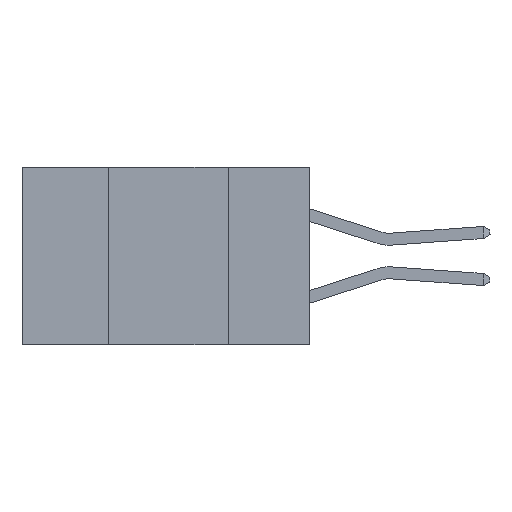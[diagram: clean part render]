
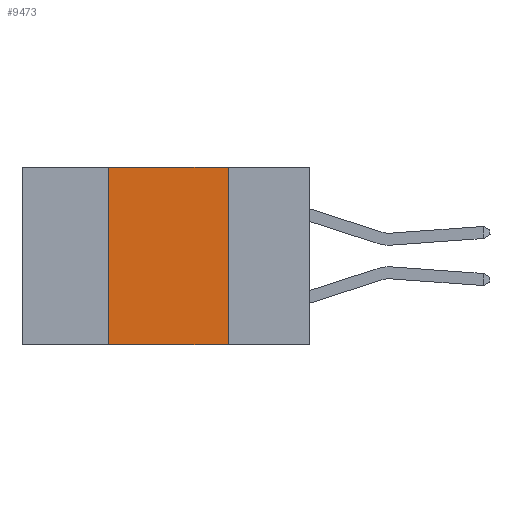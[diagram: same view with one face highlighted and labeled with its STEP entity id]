
A CAD part, left-side view. The second image highlights one B-rep face of the part: STEP entity #9473.
In plain terms, the highlighted planar face has unit normal (-1, 0, 0).
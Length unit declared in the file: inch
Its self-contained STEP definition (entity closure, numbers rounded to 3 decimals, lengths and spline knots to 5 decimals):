
#1128 = VECTOR ( 'NONE', #13885, 39.37008 ) ;
#2128 = CARTESIAN_POINT ( 'NONE',  ( 0., 0.6, 0. ) ) ;
#2676 = DIRECTION ( 'NONE',  ( 0., -1., 0. ) ) ;
#3066 = CARTESIAN_POINT ( 'NONE',  ( 0., 0.6, 0. ) ) ;
#3781 = VERTEX_POINT ( 'NONE', #9034 ) ;
#5067 = FACE_OUTER_BOUND ( 'NONE', #28267, .T. ) ;
#5304 = VERTEX_POINT ( 'NONE', #15495 ) ;
#5627 = LINE ( 'NONE', #27259, #1128 ) ;
#6877 = DIRECTION ( 'NONE',  ( 1., 0., 0. ) ) ;
#7494 = LINE ( 'NONE', #3066, #9199 ) ;
#9034 = CARTESIAN_POINT ( 'NONE',  ( 0., 0.42, 0. ) ) ;
#9103 = CARTESIAN_POINT ( 'NONE',  ( 0., 0.17, 0. ) ) ;
#9199 = VECTOR ( 'NONE', #2676, 39.37008 ) ;
#9473 = ADVANCED_FACE ( 'NONE', ( #5067 ), #11490, .F. ) ;
#10404 = ORIENTED_EDGE ( 'NONE', *, *, #20025, .F. ) ;
#11490 = PLANE ( 'NONE',  #12974 ) ;
#12974 = AXIS2_PLACEMENT_3D ( 'NONE', #2128, #6877, #27038 ) ;
#13355 = LINE ( 'NONE', #9103, #26652 ) ;
#13885 = DIRECTION ( 'NONE',  ( 0., 0., 1. ) ) ;
#15495 = CARTESIAN_POINT ( 'NONE',  ( 0., 0.17, 0. ) ) ;
#18229 = EDGE_CURVE ( 'NONE', #3781, #5304, #7494, .T. ) ;
#18566 = LINE ( 'NONE', #24984, #23104 ) ;
#18690 = CARTESIAN_POINT ( 'NONE',  ( 0., 0.42, -0.37 ) ) ;
#18748 = ORIENTED_EDGE ( 'NONE', *, *, #18229, .F. ) ;
#19808 = CARTESIAN_POINT ( 'NONE',  ( 0., 0.17, -0.37 ) ) ;
#20025 = EDGE_CURVE ( 'NONE', #5304, #22705, #13355, .T. ) ;
#22705 = VERTEX_POINT ( 'NONE', #19808 ) ;
#22988 = EDGE_CURVE ( 'NONE', #24951, #22705, #18566, .T. ) ;
#23104 = VECTOR ( 'NONE', #25170, 39.37008 ) ;
#23361 = EDGE_CURVE ( 'NONE', #24951, #3781, #5627, .T. ) ;
#24951 = VERTEX_POINT ( 'NONE', #18690 ) ;
#24984 = CARTESIAN_POINT ( 'NONE',  ( 0., 0.6, -0.37 ) ) ;
#25115 = ORIENTED_EDGE ( 'NONE', *, *, #22988, .T. ) ;
#25170 = DIRECTION ( 'NONE',  ( 0., -1., 0. ) ) ;
#26148 = ORIENTED_EDGE ( 'NONE', *, *, #23361, .F. ) ;
#26652 = VECTOR ( 'NONE', #26739, 39.37008 ) ;
#26739 = DIRECTION ( 'NONE',  ( 0., 0., -1. ) ) ;
#27038 = DIRECTION ( 'NONE',  ( 0., 0., -1. ) ) ;
#27259 = CARTESIAN_POINT ( 'NONE',  ( 0., 0.42, 0. ) ) ;
#28267 = EDGE_LOOP ( 'NONE', ( #10404, #18748, #26148, #25115 ) ) ;
